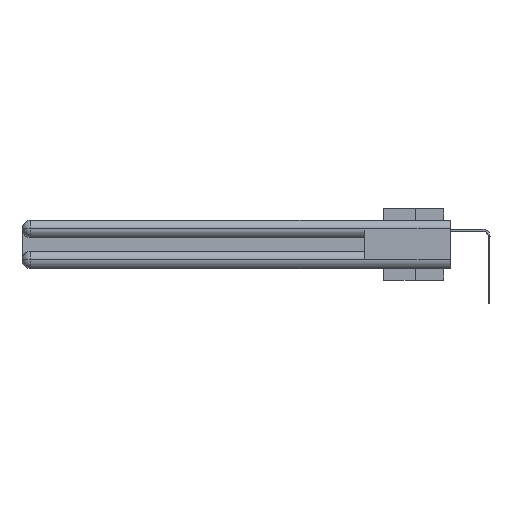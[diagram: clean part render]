
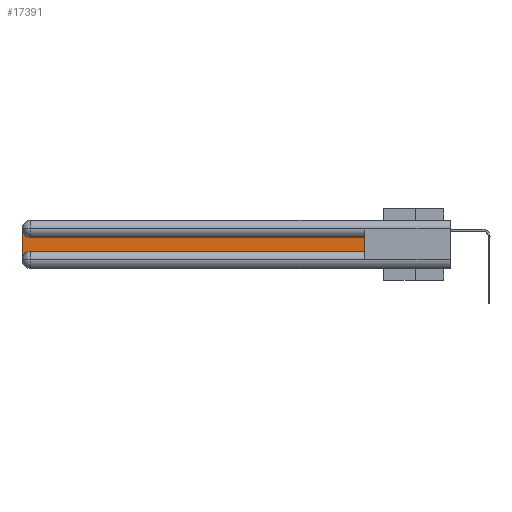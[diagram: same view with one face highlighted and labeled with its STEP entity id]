
A CAD part, left-side view. The second image highlights one B-rep face of the part: STEP entity #17391.
In plain terms, the highlighted planar face has unit normal (-1, 0, 0).
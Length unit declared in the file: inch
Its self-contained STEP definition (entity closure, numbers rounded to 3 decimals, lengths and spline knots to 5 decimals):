
#975 = VECTOR ( 'NONE', #16760, 39.37008 ) ;
#2421 = DIRECTION ( 'NONE',  ( 0., 0., -1. ) ) ;
#2668 = ORIENTED_EDGE ( 'NONE', *, *, #18562, .T. ) ;
#3143 = VERTEX_POINT ( 'NONE', #11944 ) ;
#3959 = CARTESIAN_POINT ( 'NONE',  ( 0.075, 3., -0.0625 ) ) ;
#4315 = VERTEX_POINT ( 'NONE', #33533 ) ;
#4346 = DIRECTION ( 'NONE',  ( 0., 0., 1. ) ) ;
#4601 = LINE ( 'NONE', #6820, #25381 ) ;
#5005 = LINE ( 'NONE', #8077, #15191 ) ;
#5500 = EDGE_CURVE ( 'NONE', #7629, #28772, #4601, .T. ) ;
#5549 = AXIS2_PLACEMENT_3D ( 'NONE', #8651, #25020, #11387 ) ;
#5766 = AXIS2_PLACEMENT_3D ( 'NONE', #25964, #12210, #20859 ) ;
#6382 = EDGE_CURVE ( 'NONE', #18779, #4315, #5005, .T. ) ;
#6817 = EDGE_CURVE ( 'NONE', #4315, #3143, #15602, .T. ) ;
#6820 = CARTESIAN_POINT ( 'NONE',  ( 0.075, 0.6, -0.2175 ) ) ;
#7384 = FACE_OUTER_BOUND ( 'NONE', #20170, .T. ) ;
#7629 = VERTEX_POINT ( 'NONE', #13229 ) ;
#8077 = CARTESIAN_POINT ( 'NONE',  ( 0.075, 3., -0.2175 ) ) ;
#8480 = DIRECTION ( 'NONE',  ( 0., 1., 0. ) ) ;
#8651 = CARTESIAN_POINT ( 'NONE',  ( 0.075, 3., -0.1225 ) ) ;
#11387 = DIRECTION ( 'NONE',  ( 0., 0., -1. ) ) ;
#11535 = EDGE_CURVE ( 'NONE', #28772, #24408, #18778, .T. ) ;
#11944 = CARTESIAN_POINT ( 'NONE',  ( 0.075, 2.94, -0.2175 ) ) ;
#12206 = ORIENTED_EDGE ( 'NONE', *, *, #11535, .T. ) ;
#12210 = DIRECTION ( 'NONE',  ( 1., 0., 0. ) ) ;
#13229 = CARTESIAN_POINT ( 'NONE',  ( 0.075, 0.6, -0.2175 ) ) ;
#13536 = DIRECTION ( 'NONE',  ( 0., 0., -1. ) ) ;
#13690 = EDGE_CURVE ( 'NONE', #24408, #18779, #16918, .T. ) ;
#14110 = CARTESIAN_POINT ( 'NONE',  ( 0.075, 0.6, -0.1225 ) ) ;
#15039 = ORIENTED_EDGE ( 'NONE', *, *, #5500, .T. ) ;
#15191 = VECTOR ( 'NONE', #13536, 39.37008 ) ;
#15558 = ORIENTED_EDGE ( 'NONE', *, *, #6817, .T. ) ;
#15602 = CIRCLE ( 'NONE', #5766, 0.06 ) ;
#16760 = DIRECTION ( 'NONE',  ( 0., -1., 0. ) ) ;
#16918 = CIRCLE ( 'NONE', #31065, 0.06 ) ;
#17391 = ADVANCED_FACE ( 'NONE', ( #7384 ), #24891, .F. ) ;
#18562 = EDGE_CURVE ( 'NONE', #3143, #7629, #27214, .T. ) ;
#18658 = CARTESIAN_POINT ( 'NONE',  ( 0.075, 2.94, -0.0625 ) ) ;
#18778 = LINE ( 'NONE', #24946, #27245 ) ;
#18779 = VERTEX_POINT ( 'NONE', #3959 ) ;
#20170 = EDGE_LOOP ( 'NONE', ( #12206, #32691, #31254, #15558, #2668, #15039 ) ) ;
#20859 = DIRECTION ( 'NONE',  ( 0., 0., -1. ) ) ;
#24408 = VERTEX_POINT ( 'NONE', #30016 ) ;
#24891 = PLANE ( 'NONE',  #5549 ) ;
#24946 = CARTESIAN_POINT ( 'NONE',  ( 0.075, 0.6, -0.1225 ) ) ;
#25020 = DIRECTION ( 'NONE',  ( 1., 0., 0. ) ) ;
#25297 = CARTESIAN_POINT ( 'NONE',  ( 0.075, 0.6, -0.2175 ) ) ;
#25381 = VECTOR ( 'NONE', #4346, 39.37008 ) ;
#25964 = CARTESIAN_POINT ( 'NONE',  ( 0.075, 2.94, -0.2775 ) ) ;
#26465 = DIRECTION ( 'NONE',  ( 1., 0., 0. ) ) ;
#27214 = LINE ( 'NONE', #25297, #975 ) ;
#27245 = VECTOR ( 'NONE', #8480, 39.37008 ) ;
#28772 = VERTEX_POINT ( 'NONE', #14110 ) ;
#30016 = CARTESIAN_POINT ( 'NONE',  ( 0.075, 2.94, -0.1225 ) ) ;
#31065 = AXIS2_PLACEMENT_3D ( 'NONE', #18658, #26465, #2421 ) ;
#31254 = ORIENTED_EDGE ( 'NONE', *, *, #6382, .T. ) ;
#32691 = ORIENTED_EDGE ( 'NONE', *, *, #13690, .T. ) ;
#33533 = CARTESIAN_POINT ( 'NONE',  ( 0.075, 3., -0.2775 ) ) ;
